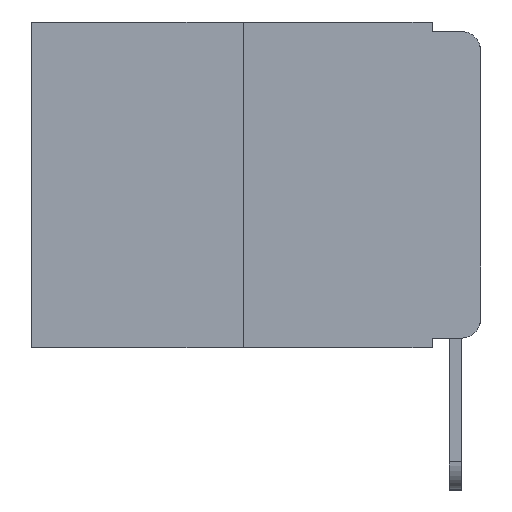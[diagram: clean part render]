
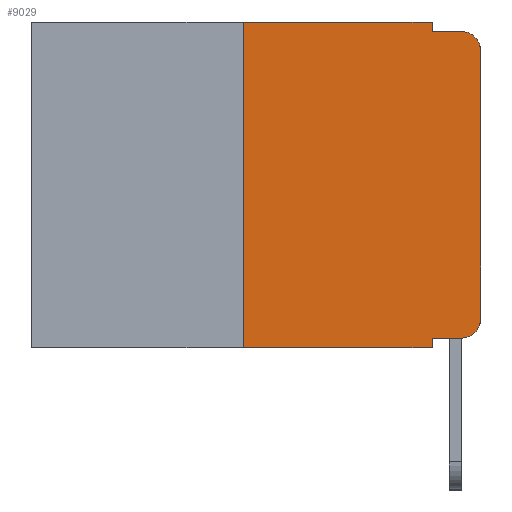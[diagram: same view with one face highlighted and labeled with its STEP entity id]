
A CAD part, left-side view. The second image highlights one B-rep face of the part: STEP entity #9029.
In plain terms, the highlighted planar face has unit normal (-1, 0, 0).
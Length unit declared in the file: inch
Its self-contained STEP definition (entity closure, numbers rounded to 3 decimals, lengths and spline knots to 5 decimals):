
#315 = VERTEX_POINT ( 'NONE', #2619 ) ;
#426 = CARTESIAN_POINT ( 'NONE',  ( 0., 0., 0. ) ) ;
#640 = ORIENTED_EDGE ( 'NONE', *, *, #10212, .F. ) ;
#657 = ORIENTED_EDGE ( 'NONE', *, *, #10419, .F. ) ;
#666 = ORIENTED_EDGE ( 'NONE', *, *, #7097, .F. ) ;
#811 = DIRECTION ( 'NONE',  ( -1., 0., 0. ) ) ;
#824 = CARTESIAN_POINT ( 'NONE',  ( 0., 0.02, -0.313 ) ) ;
#975 = ORIENTED_EDGE ( 'NONE', *, *, #4563, .T. ) ;
#1011 = ORIENTED_EDGE ( 'NONE', *, *, #3305, .T. ) ;
#1433 = LINE ( 'NONE', #10289, #6367 ) ;
#1537 = CARTESIAN_POINT ( 'NONE',  ( 0., 0.051, -0.333 ) ) ;
#1548 = DIRECTION ( 'NONE',  ( 0., -1., 0. ) ) ;
#1597 = VECTOR ( 'NONE', #1548, 39.37008 ) ;
#1648 = DIRECTION ( 'NONE',  ( 0., -1., 0. ) ) ;
#1842 = EDGE_CURVE ( 'NONE', #2755, #2112, #8158, .T. ) ;
#2112 = VERTEX_POINT ( 'NONE', #5897 ) ;
#2216 = LINE ( 'NONE', #4510, #1597 ) ;
#2325 = VECTOR ( 'NONE', #1648, 39.37008 ) ;
#2619 = CARTESIAN_POINT ( 'NONE',  ( 0., 0.051, 0. ) ) ;
#2755 = VERTEX_POINT ( 'NONE', #10563 ) ;
#2786 = VERTEX_POINT ( 'NONE', #10950 ) ;
#2806 = AXIS2_PLACEMENT_3D ( 'NONE', #824, #811, #10184 ) ;
#2845 = VERTEX_POINT ( 'NONE', #8144 ) ;
#2880 = DIRECTION ( 'NONE',  ( 1., 0., 0. ) ) ;
#2915 = FACE_OUTER_BOUND ( 'NONE', #8229, .T. ) ;
#3021 = VECTOR ( 'NONE', #6960, 39.37008 ) ;
#3158 = DIRECTION ( 'NONE',  ( 0., 0., -1. ) ) ;
#3206 = AXIS2_PLACEMENT_3D ( 'NONE', #5873, #2880, #5947 ) ;
#3305 = EDGE_CURVE ( 'NONE', #9070, #8689, #5898, .T. ) ;
#3313 = VECTOR ( 'NONE', #3665, 39.37008 ) ;
#3377 = CARTESIAN_POINT ( 'NONE',  ( 0., 0.25, -0.343 ) ) ;
#3665 = DIRECTION ( 'NONE',  ( 0., 0., 1. ) ) ;
#4063 = EDGE_CURVE ( 'NONE', #7192, #2112, #5150, .T. ) ;
#4405 = DIRECTION ( 'NONE',  ( 0., 0., 1. ) ) ;
#4459 = CARTESIAN_POINT ( 'NONE',  ( 0., 0.25, 0. ) ) ;
#4510 = CARTESIAN_POINT ( 'NONE',  ( 0., 0.473, 0. ) ) ;
#4563 = EDGE_CURVE ( 'NONE', #8689, #11946, #7348, .T. ) ;
#4902 = ORIENTED_EDGE ( 'NONE', *, *, #4063, .T. ) ;
#5007 = LINE ( 'NONE', #1537, #2325 ) ;
#5083 = DIRECTION ( 'NONE',  ( -1., 0., 0. ) ) ;
#5150 = LINE ( 'NONE', #7223, #9869 ) ;
#5731 = AXIS2_PLACEMENT_3D ( 'NONE', #6983, #5083, #9036 ) ;
#5779 = CARTESIAN_POINT ( 'NONE',  ( 0., 0., -0.03 ) ) ;
#5836 = CARTESIAN_POINT ( 'NONE',  ( 0., 0., -0.313 ) ) ;
#5840 = EDGE_CURVE ( 'NONE', #7192, #8894, #9988, .T. ) ;
#5873 = CARTESIAN_POINT ( 'NONE',  ( 0., 0.473, 0. ) ) ;
#5897 = CARTESIAN_POINT ( 'NONE',  ( 0., 0.051, -0.343 ) ) ;
#5898 = LINE ( 'NONE', #426, #3313 ) ;
#5947 = DIRECTION ( 'NONE',  ( 0., 0., -1. ) ) ;
#6067 = CIRCLE ( 'NONE', #2806, 0.02 ) ;
#6362 = ORIENTED_EDGE ( 'NONE', *, *, #12342, .T. ) ;
#6367 = VECTOR ( 'NONE', #10277, 39.37008 ) ;
#6960 = DIRECTION ( 'NONE',  ( 0., 0., -1. ) ) ;
#6983 = CARTESIAN_POINT ( 'NONE',  ( 0., 0.02, -0.03 ) ) ;
#7097 = EDGE_CURVE ( 'NONE', #315, #2786, #11806, .T. ) ;
#7192 = VERTEX_POINT ( 'NONE', #3377 ) ;
#7223 = CARTESIAN_POINT ( 'NONE',  ( 0., 0.473, -0.343 ) ) ;
#7348 = CIRCLE ( 'NONE', #5731, 0.02 ) ;
#8144 = CARTESIAN_POINT ( 'NONE',  ( 0., 0.02, -0.333 ) ) ;
#8158 = LINE ( 'NONE', #10541, #3021 ) ;
#8182 = DIRECTION ( 'NONE',  ( 0., -1., 0. ) ) ;
#8229 = EDGE_LOOP ( 'NONE', ( #1011, #975, #640, #666, #657, #9040, #4902, #10217, #6362, #8607 ) ) ;
#8445 = CARTESIAN_POINT ( 'NONE',  ( 0., 0.051, 0. ) ) ;
#8564 = CARTESIAN_POINT ( 'NONE',  ( 0., 0.02, -0.01 ) ) ;
#8607 = ORIENTED_EDGE ( 'NONE', *, *, #11128, .T. ) ;
#8657 = PLANE ( 'NONE',  #3206 ) ;
#8689 = VERTEX_POINT ( 'NONE', #5779 ) ;
#8815 = CARTESIAN_POINT ( 'NONE',  ( 0., 0.25, 0. ) ) ;
#8894 = VERTEX_POINT ( 'NONE', #4459 ) ;
#9029 = ADVANCED_FACE ( 'NONE', ( #2915 ), #8657, .F. ) ;
#9036 = DIRECTION ( 'NONE',  ( 0., 0., -1. ) ) ;
#9040 = ORIENTED_EDGE ( 'NONE', *, *, #5840, .F. ) ;
#9068 = VECTOR ( 'NONE', #3158, 39.37008 ) ;
#9070 = VERTEX_POINT ( 'NONE', #5836 ) ;
#9869 = VECTOR ( 'NONE', #8182, 39.37008 ) ;
#9988 = LINE ( 'NONE', #8815, #12137 ) ;
#10184 = DIRECTION ( 'NONE',  ( 0., 0., -1. ) ) ;
#10212 = EDGE_CURVE ( 'NONE', #2786, #11946, #1433, .T. ) ;
#10217 = ORIENTED_EDGE ( 'NONE', *, *, #1842, .F. ) ;
#10277 = DIRECTION ( 'NONE',  ( 0., -1., 0. ) ) ;
#10289 = CARTESIAN_POINT ( 'NONE',  ( 0., 0.051, -0.01 ) ) ;
#10419 = EDGE_CURVE ( 'NONE', #8894, #315, #2216, .T. ) ;
#10541 = CARTESIAN_POINT ( 'NONE',  ( 0., 0.051, 0. ) ) ;
#10563 = CARTESIAN_POINT ( 'NONE',  ( 0., 0.051, -0.333 ) ) ;
#10950 = CARTESIAN_POINT ( 'NONE',  ( 0., 0.051, -0.01 ) ) ;
#11128 = EDGE_CURVE ( 'NONE', #2845, #9070, #6067, .T. ) ;
#11806 = LINE ( 'NONE', #8445, #9068 ) ;
#11946 = VERTEX_POINT ( 'NONE', #8564 ) ;
#12137 = VECTOR ( 'NONE', #4405, 39.37008 ) ;
#12342 = EDGE_CURVE ( 'NONE', #2755, #2845, #5007, .T. ) ;
